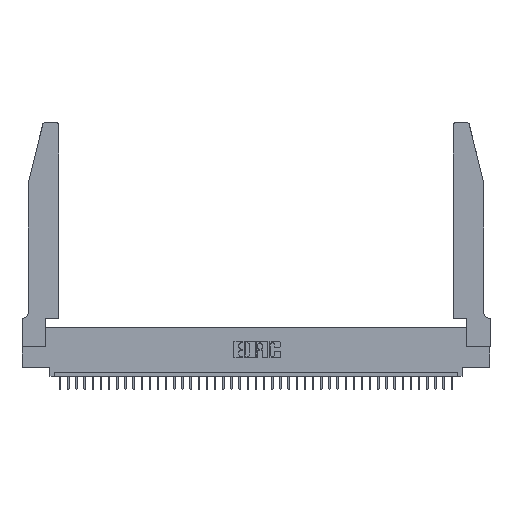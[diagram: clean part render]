
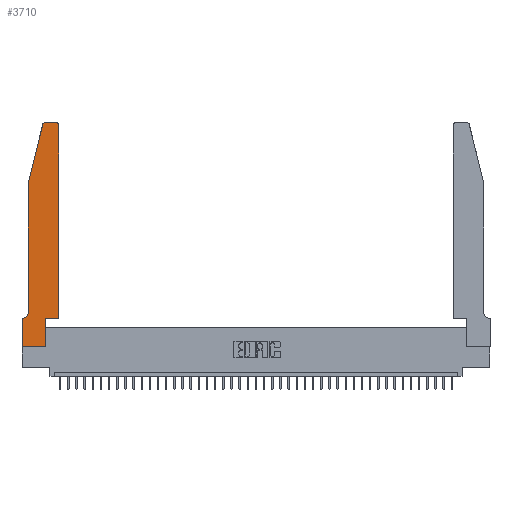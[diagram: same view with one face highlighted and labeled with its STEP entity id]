
A CAD part, top view. The second image highlights one B-rep face of the part: STEP entity #3710.
In plain terms, the highlighted planar face has unit normal (0, 0, 1).
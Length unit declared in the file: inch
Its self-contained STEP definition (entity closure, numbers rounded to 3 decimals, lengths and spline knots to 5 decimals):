
#251 = CARTESIAN_POINT ( 'NONE',  ( 0., 0.35, 0.37 ) ) ;
#514 = CARTESIAN_POINT ( 'NONE',  ( 0.0755, 2., 0.37 ) ) ;
#652 = EDGE_CURVE ( 'NONE', #6507, #21767, #5785, .T. ) ;
#1062 = VERTEX_POINT ( 'NONE', #13984 ) ;
#1299 = EDGE_CURVE ( 'NONE', #33700, #16054, #38251, .T. ) ;
#2396 = ORIENTED_EDGE ( 'NONE', *, *, #11945, .T. ) ;
#2735 = VERTEX_POINT ( 'NONE', #31529 ) ;
#2749 = VERTEX_POINT ( 'NONE', #16131 ) ;
#2774 = CARTESIAN_POINT ( 'NONE',  ( 0.0055, 0.35, 0.37 ) ) ;
#2976 = CARTESIAN_POINT ( 'NONE',  ( 0., 0., 0.37 ) ) ;
#3259 = CARTESIAN_POINT ( 'NONE',  ( 0., 0., 0.37 ) ) ;
#3481 = LINE ( 'NONE', #11265, #22675 ) ;
#3561 = DIRECTION ( 'NONE',  ( 1., 0., 0. ) ) ;
#3710 = ADVANCED_FACE ( 'NONE', ( #38486 ), #6227, .T. ) ;
#4044 = LINE ( 'NONE', #14394, #35101 ) ;
#4526 = ORIENTED_EDGE ( 'NONE', *, *, #22169, .T. ) ;
#4571 = ORIENTED_EDGE ( 'NONE', *, *, #7698, .T. ) ;
#4801 = VECTOR ( 'NONE', #33483, 39.37008 ) ;
#5236 = VERTEX_POINT ( 'NONE', #13698 ) ;
#5785 = LINE ( 'NONE', #22593, #4801 ) ;
#5927 = EDGE_CURVE ( 'NONE', #6046, #2735, #40922, .T. ) ;
#6046 = VERTEX_POINT ( 'NONE', #8103 ) ;
#6053 = ORIENTED_EDGE ( 'NONE', *, *, #9860, .T. ) ;
#6227 = PLANE ( 'NONE',  #34019 ) ;
#6396 = CARTESIAN_POINT ( 'NONE',  ( 0.4205, 2.72, 0.37 ) ) ;
#6507 = VERTEX_POINT ( 'NONE', #2774 ) ;
#6522 = DIRECTION ( 'NONE',  ( 0., 0., 1. ) ) ;
#6736 = CARTESIAN_POINT ( 'NONE',  ( 0.284, 2.72, 0.37 ) ) ;
#6847 = CARTESIAN_POINT ( 'NONE',  ( 0.2865, 0.35, 0.37 ) ) ;
#7016 = DIRECTION ( 'NONE',  ( 0., 0., 1. ) ) ;
#7698 = EDGE_CURVE ( 'NONE', #21767, #24721, #10478, .T. ) ;
#8103 = CARTESIAN_POINT ( 'NONE',  ( 0.4505, 2.72, 0.37 ) ) ;
#8458 = DIRECTION ( 'NONE',  ( 0., 1., 0. ) ) ;
#8883 = EDGE_CURVE ( 'NONE', #5236, #22048, #4044, .T. ) ;
#8888 = AXIS2_PLACEMENT_3D ( 'NONE', #33907, #18289, #24617 ) ;
#9860 = EDGE_CURVE ( 'NONE', #24721, #36536, #13229, .T. ) ;
#10046 = AXIS2_PLACEMENT_3D ( 'NONE', #6736, #7016, #13037 ) ;
#10478 = LINE ( 'NONE', #2976, #40211 ) ;
#11135 = DIRECTION ( 'NONE',  ( -1., 0., 0. ) ) ;
#11265 = CARTESIAN_POINT ( 'NONE',  ( 0.4505, 0.35, 0.37 ) ) ;
#11342 = CARTESIAN_POINT ( 'NONE',  ( 0.2865, 0.35, 0.37 ) ) ;
#11945 = EDGE_CURVE ( 'NONE', #36536, #33700, #26970, .T. ) ;
#12587 = DIRECTION ( 'NONE',  ( 1., 0., 0. ) ) ;
#13037 = DIRECTION ( 'NONE',  ( 1., 0., 0. ) ) ;
#13229 = LINE ( 'NONE', #22807, #40057 ) ;
#13425 = DIRECTION ( 'NONE',  ( 1., 0., 0. ) ) ;
#13698 = CARTESIAN_POINT ( 'NONE',  ( 0.25487, 2.72718, 0.37 ) ) ;
#13984 = CARTESIAN_POINT ( 'NONE',  ( 0.0755, 0.42, 0.37 ) ) ;
#14286 = DIRECTION ( 'NONE',  ( 1., 0., 0. ) ) ;
#14394 = CARTESIAN_POINT ( 'NONE',  ( 0.0755, 2., 0.37 ) ) ;
#14539 = DIRECTION ( 'NONE',  ( -0.239, -0.971, 0. ) ) ;
#15207 = CARTESIAN_POINT ( 'NONE',  ( 0.2865, 0., 0.37 ) ) ;
#16054 = VERTEX_POINT ( 'NONE', #20941 ) ;
#16131 = CARTESIAN_POINT ( 'NONE',  ( 0.284, 2.75, 0.37 ) ) ;
#16245 = EDGE_CURVE ( 'NONE', #1062, #6507, #24198, .T. ) ;
#17117 = VECTOR ( 'NONE', #40224, 39.37008 ) ;
#18289 = DIRECTION ( 'NONE',  ( 0., 0., -1. ) ) ;
#18363 = CARTESIAN_POINT ( 'NONE',  ( 0., 0.35, 0.37 ) ) ;
#18945 = DIRECTION ( 'NONE',  ( 0., -1., 0. ) ) ;
#20063 = CARTESIAN_POINT ( 'NONE',  ( 0.4505, 0.35, 0.37 ) ) ;
#20941 = CARTESIAN_POINT ( 'NONE',  ( 0.4505, 0.35, 0.37 ) ) ;
#21556 = EDGE_CURVE ( 'NONE', #22048, #1062, #22494, .T. ) ;
#21767 = VERTEX_POINT ( 'NONE', #18363 ) ;
#22006 = VECTOR ( 'NONE', #8458, 39.37008 ) ;
#22048 = VERTEX_POINT ( 'NONE', #514 ) ;
#22169 = EDGE_CURVE ( 'NONE', #2735, #2749, #33458, .T. ) ;
#22494 = LINE ( 'NONE', #24593, #17117 ) ;
#22593 = CARTESIAN_POINT ( 'NONE',  ( 0.0755, 0.35, 0.37 ) ) ;
#22675 = VECTOR ( 'NONE', #23850, 39.37008 ) ;
#22807 = CARTESIAN_POINT ( 'NONE',  ( 0., 0., 0.37 ) ) ;
#23277 = CIRCLE ( 'NONE', #10046, 0.03 ) ;
#23850 = DIRECTION ( 'NONE',  ( 0., 1., 0. ) ) ;
#24026 = ORIENTED_EDGE ( 'NONE', *, *, #8883, .T. ) ;
#24198 = CIRCLE ( 'NONE', #8888, 0.07 ) ;
#24593 = CARTESIAN_POINT ( 'NONE',  ( 0.0755, 2., 0.37 ) ) ;
#24617 = DIRECTION ( 'NONE',  ( -1., 0., 0. ) ) ;
#24721 = VERTEX_POINT ( 'NONE', #3259 ) ;
#25204 = EDGE_CURVE ( 'NONE', #2749, #5236, #23277, .T. ) ;
#26970 = LINE ( 'NONE', #11342, #22006 ) ;
#28220 = EDGE_LOOP ( 'NONE', ( #4526, #28903, #24026, #28940, #34292, #38925, #4571, #6053, #2396, #34800, #30663, #37479 ) ) ;
#28903 = ORIENTED_EDGE ( 'NONE', *, *, #25204, .T. ) ;
#28940 = ORIENTED_EDGE ( 'NONE', *, *, #21556, .T. ) ;
#29912 = VECTOR ( 'NONE', #14286, 39.37008 ) ;
#30663 = ORIENTED_EDGE ( 'NONE', *, *, #39279, .T. ) ;
#31529 = CARTESIAN_POINT ( 'NONE',  ( 0.4205, 2.75, 0.37 ) ) ;
#31860 = DIRECTION ( 'NONE',  ( 0., 0., 1. ) ) ;
#32904 = VECTOR ( 'NONE', #11135, 39.37008 ) ;
#32980 = CARTESIAN_POINT ( 'NONE',  ( 0.2605, 2.75, 0.37 ) ) ;
#33458 = LINE ( 'NONE', #32980, #32904 ) ;
#33483 = DIRECTION ( 'NONE',  ( -1., 0., 0. ) ) ;
#33700 = VERTEX_POINT ( 'NONE', #6847 ) ;
#33907 = CARTESIAN_POINT ( 'NONE',  ( 0.0055, 0.42, 0.37 ) ) ;
#34019 = AXIS2_PLACEMENT_3D ( 'NONE', #251, #31860, #3561 ) ;
#34292 = ORIENTED_EDGE ( 'NONE', *, *, #16245, .T. ) ;
#34800 = ORIENTED_EDGE ( 'NONE', *, *, #1299, .T. ) ;
#35101 = VECTOR ( 'NONE', #14539, 39.37008 ) ;
#36536 = VERTEX_POINT ( 'NONE', #15207 ) ;
#37479 = ORIENTED_EDGE ( 'NONE', *, *, #5927, .T. ) ;
#37723 = AXIS2_PLACEMENT_3D ( 'NONE', #6396, #6522, #12587 ) ;
#38251 = LINE ( 'NONE', #20063, #29912 ) ;
#38486 = FACE_OUTER_BOUND ( 'NONE', #28220, .T. ) ;
#38925 = ORIENTED_EDGE ( 'NONE', *, *, #652, .T. ) ;
#39279 = EDGE_CURVE ( 'NONE', #16054, #6046, #3481, .T. ) ;
#40057 = VECTOR ( 'NONE', #13425, 39.37008 ) ;
#40211 = VECTOR ( 'NONE', #18945, 39.37008 ) ;
#40224 = DIRECTION ( 'NONE',  ( 0., -1., 0. ) ) ;
#40922 = CIRCLE ( 'NONE', #37723, 0.03 ) ;
